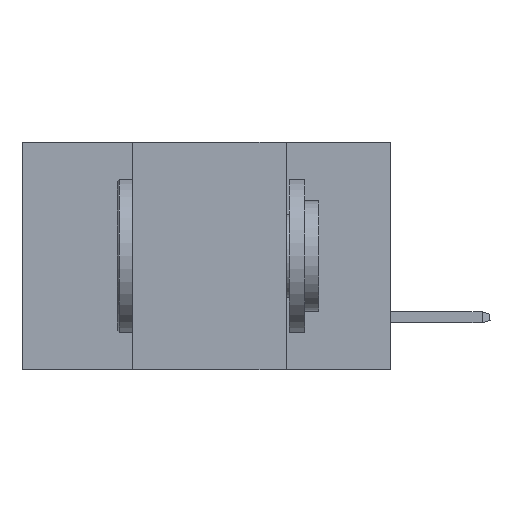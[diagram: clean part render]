
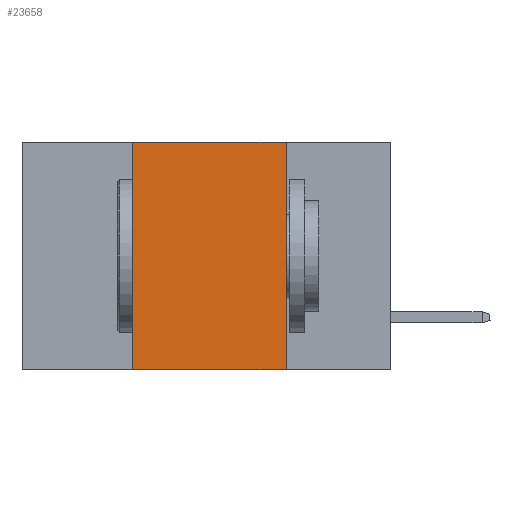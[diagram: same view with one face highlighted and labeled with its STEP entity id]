
A CAD part, left-side view. The second image highlights one B-rep face of the part: STEP entity #23658.
In plain terms, the highlighted planar face has unit normal (-1, 0, 0).
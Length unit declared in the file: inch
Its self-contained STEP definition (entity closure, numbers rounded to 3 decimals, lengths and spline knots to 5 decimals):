
#3584 = CARTESIAN_POINT ( 'NONE',  ( 0., 0.6, 0. ) ) ;
#3704 = LINE ( 'NONE', #16475, #19873 ) ;
#5288 = VERTEX_POINT ( 'NONE', #28961 ) ;
#6216 = DIRECTION ( 'NONE',  ( 1., 0., 0. ) ) ;
#7297 = AXIS2_PLACEMENT_3D ( 'NONE', #19208, #6216, #25234 ) ;
#7339 = ORIENTED_EDGE ( 'NONE', *, *, #22280, .T. ) ;
#10213 = DIRECTION ( 'NONE',  ( 0., 0., -1. ) ) ;
#16475 = CARTESIAN_POINT ( 'NONE',  ( 0., 0.17, 0. ) ) ;
#17101 = CARTESIAN_POINT ( 'NONE',  ( 0., 0.42, 0. ) ) ;
#17336 = ORIENTED_EDGE ( 'NONE', *, *, #22034, .F. ) ;
#17728 = FACE_OUTER_BOUND ( 'NONE', #27399, .T. ) ;
#19080 = PLANE ( 'NONE',  #7297 ) ;
#19208 = CARTESIAN_POINT ( 'NONE',  ( 0., 0.6, 0. ) ) ;
#19873 = VECTOR ( 'NONE', #10213, 39.37008 ) ;
#20634 = CARTESIAN_POINT ( 'NONE',  ( 0., 0.6, -0.37 ) ) ;
#22034 = EDGE_CURVE ( 'NONE', #34499, #31248, #3704, .T. ) ;
#22112 = LINE ( 'NONE', #17101, #33620 ) ;
#22280 = EDGE_CURVE ( 'NONE', #5288, #31248, #37907, .T. ) ;
#23658 = ADVANCED_FACE ( 'NONE', ( #17728 ), #19080, .F. ) ;
#24679 = CARTESIAN_POINT ( 'NONE',  ( 0., 0.17, 0. ) ) ;
#24774 = ORIENTED_EDGE ( 'NONE', *, *, #29333, .F. ) ;
#25234 = DIRECTION ( 'NONE',  ( 0., 0., -1. ) ) ;
#27399 = EDGE_LOOP ( 'NONE', ( #17336, #24774, #36532, #7339 ) ) ;
#28961 = CARTESIAN_POINT ( 'NONE',  ( 0., 0.42, -0.37 ) ) ;
#29333 = EDGE_CURVE ( 'NONE', #37188, #34499, #39388, .T. ) ;
#30805 = VECTOR ( 'NONE', #32808, 39.37008 ) ;
#30853 = CARTESIAN_POINT ( 'NONE',  ( 0., 0.42, 0. ) ) ;
#30945 = DIRECTION ( 'NONE',  ( 0., -1., 0. ) ) ;
#31248 = VERTEX_POINT ( 'NONE', #37976 ) ;
#32808 = DIRECTION ( 'NONE',  ( 0., -1., 0. ) ) ;
#33620 = VECTOR ( 'NONE', #35757, 39.37008 ) ;
#34499 = VERTEX_POINT ( 'NONE', #24679 ) ;
#35757 = DIRECTION ( 'NONE',  ( 0., 0., 1. ) ) ;
#36532 = ORIENTED_EDGE ( 'NONE', *, *, #40456, .F. ) ;
#37188 = VERTEX_POINT ( 'NONE', #30853 ) ;
#37907 = LINE ( 'NONE', #20634, #38911 ) ;
#37976 = CARTESIAN_POINT ( 'NONE',  ( 0., 0.17, -0.37 ) ) ;
#38911 = VECTOR ( 'NONE', #30945, 39.37008 ) ;
#39388 = LINE ( 'NONE', #3584, #30805 ) ;
#40456 = EDGE_CURVE ( 'NONE', #5288, #37188, #22112, .T. ) ;
